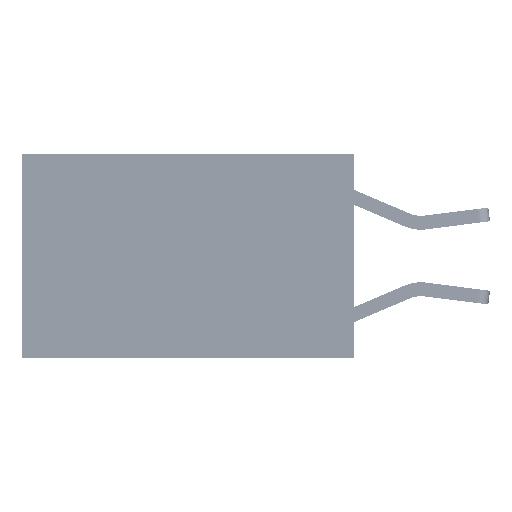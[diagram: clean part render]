
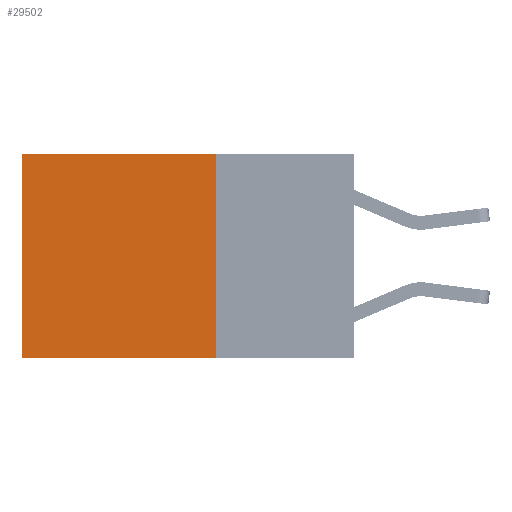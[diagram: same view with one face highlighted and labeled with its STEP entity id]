
A CAD part, left-side view. The second image highlights one B-rep face of the part: STEP entity #29502.
In plain terms, the highlighted planar face has unit normal (-1, 0, 0).
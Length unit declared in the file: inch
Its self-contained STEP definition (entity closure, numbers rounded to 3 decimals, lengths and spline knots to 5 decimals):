
#35 = LINE ( 'NONE', #6125, #5734 ) ;
#1031 = PLANE ( 'NONE',  #2204 ) ;
#2186 = EDGE_LOOP ( 'NONE', ( #16036, #12951, #5770, #10815 ) ) ;
#2204 = AXIS2_PLACEMENT_3D ( 'NONE', #20497, #30294, #22900 ) ;
#2278 = DIRECTION ( 'NONE',  ( 0., 0., -1. ) ) ;
#2369 = EDGE_CURVE ( 'NONE', #25645, #11286, #13598, .T. ) ;
#2724 = CARTESIAN_POINT ( 'NONE',  ( 0.2625, 0.25, 0. ) ) ;
#5734 = VECTOR ( 'NONE', #25517, 39.37008 ) ;
#5770 = ORIENTED_EDGE ( 'NONE', *, *, #14671, .F. ) ;
#6125 = CARTESIAN_POINT ( 'NONE',  ( 0.2625, 0.25, 0. ) ) ;
#9007 = LINE ( 'NONE', #24084, #22651 ) ;
#10815 = ORIENTED_EDGE ( 'NONE', *, *, #17520, .T. ) ;
#11286 = VERTEX_POINT ( 'NONE', #27124 ) ;
#12930 = VECTOR ( 'NONE', #17398, 39.37008 ) ;
#12951 = ORIENTED_EDGE ( 'NONE', *, *, #20096, .F. ) ;
#13598 = LINE ( 'NONE', #26274, #14012 ) ;
#14012 = VECTOR ( 'NONE', #2278, 39.37008 ) ;
#14671 = EDGE_CURVE ( 'NONE', #27801, #18227, #35, .T. ) ;
#16036 = ORIENTED_EDGE ( 'NONE', *, *, #2369, .T. ) ;
#17002 = FACE_OUTER_BOUND ( 'NONE', #2186, .T. ) ;
#17398 = DIRECTION ( 'NONE',  ( 0., 1., 0. ) ) ;
#17520 = EDGE_CURVE ( 'NONE', #27801, #25645, #9007, .T. ) ;
#18227 = VERTEX_POINT ( 'NONE', #20935 ) ;
#20096 = EDGE_CURVE ( 'NONE', #18227, #11286, #24260, .T. ) ;
#20497 = CARTESIAN_POINT ( 'NONE',  ( 0.2625, 0.25, 0. ) ) ;
#20935 = CARTESIAN_POINT ( 'NONE',  ( 0.2625, 0.25, -0.37 ) ) ;
#21229 = CARTESIAN_POINT ( 'NONE',  ( 0.2625, 0.6, 0. ) ) ;
#22160 = CARTESIAN_POINT ( 'NONE',  ( 0.2625, 0.25, -0.37 ) ) ;
#22651 = VECTOR ( 'NONE', #30151, 39.37008 ) ;
#22900 = DIRECTION ( 'NONE',  ( 0., 0., -1. ) ) ;
#24084 = CARTESIAN_POINT ( 'NONE',  ( 0.2625, 0.25, 0. ) ) ;
#24260 = LINE ( 'NONE', #22160, #12930 ) ;
#25517 = DIRECTION ( 'NONE',  ( 0., 0., -1. ) ) ;
#25645 = VERTEX_POINT ( 'NONE', #21229 ) ;
#26274 = CARTESIAN_POINT ( 'NONE',  ( 0.2625, 0.6, 0. ) ) ;
#27124 = CARTESIAN_POINT ( 'NONE',  ( 0.2625, 0.6, -0.37 ) ) ;
#27801 = VERTEX_POINT ( 'NONE', #2724 ) ;
#29502 = ADVANCED_FACE ( 'NONE', ( #17002 ), #1031, .F. ) ;
#30151 = DIRECTION ( 'NONE',  ( 0., 1., 0. ) ) ;
#30294 = DIRECTION ( 'NONE',  ( 1., 0., 0. ) ) ;
